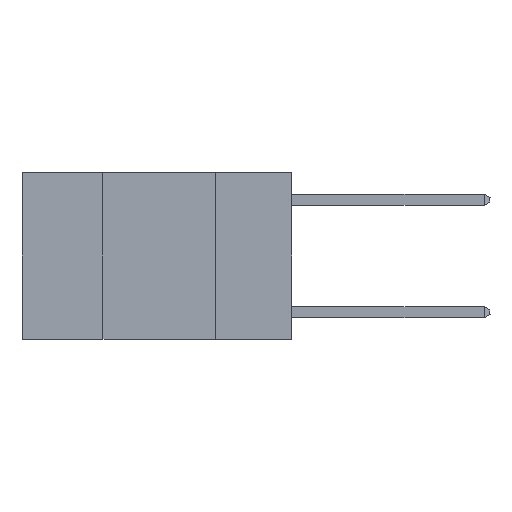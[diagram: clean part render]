
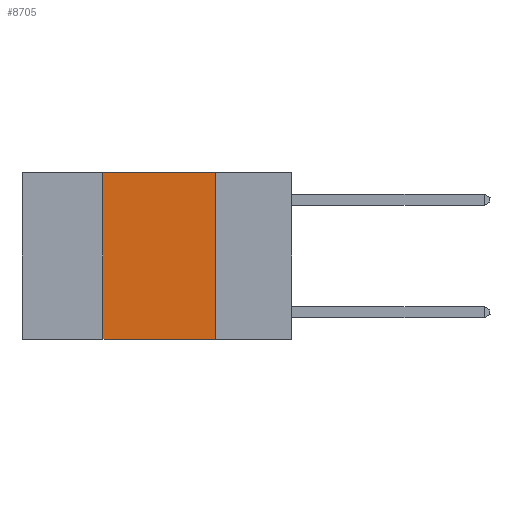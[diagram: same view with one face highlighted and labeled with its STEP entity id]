
A CAD part, left-side view. The second image highlights one B-rep face of the part: STEP entity #8705.
In plain terms, the highlighted planar face has unit normal (-1, 0, 0).
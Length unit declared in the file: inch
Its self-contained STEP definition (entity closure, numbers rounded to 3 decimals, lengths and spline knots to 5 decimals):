
#57 = VERTEX_POINT ( 'NONE', #1477 ) ;
#763 = EDGE_CURVE ( 'NONE', #57, #2991, #19208, .T. ) ;
#1477 = CARTESIAN_POINT ( 'NONE',  ( 0., 0.42, -0.37 ) ) ;
#1705 = AXIS2_PLACEMENT_3D ( 'NONE', #19868, #19673, #16497 ) ;
#2331 = ORIENTED_EDGE ( 'NONE', *, *, #6382, .T. ) ;
#2991 = VERTEX_POINT ( 'NONE', #6717 ) ;
#3141 = EDGE_LOOP ( 'NONE', ( #3991, #3973, #12207, #2331 ) ) ;
#3901 = VECTOR ( 'NONE', #5227, 39.37008 ) ;
#3973 = ORIENTED_EDGE ( 'NONE', *, *, #10713, .F. ) ;
#3991 = ORIENTED_EDGE ( 'NONE', *, *, #4081, .F. ) ;
#4081 = EDGE_CURVE ( 'NONE', #12759, #8186, #7057, .T. ) ;
#4311 = DIRECTION ( 'NONE',  ( 0., 0., -1. ) ) ;
#5227 = DIRECTION ( 'NONE',  ( 0., -1., 0. ) ) ;
#5976 = DIRECTION ( 'NONE',  ( 0., -1., 0. ) ) ;
#6382 = EDGE_CURVE ( 'NONE', #57, #8186, #9386, .T. ) ;
#6596 = VECTOR ( 'NONE', #4311, 39.37008 ) ;
#6717 = CARTESIAN_POINT ( 'NONE',  ( 0., 0.42, 0. ) ) ;
#6753 = LINE ( 'NONE', #19111, #3901 ) ;
#7057 = LINE ( 'NONE', #13520, #6596 ) ;
#8186 = VERTEX_POINT ( 'NONE', #9035 ) ;
#8705 = ADVANCED_FACE ( 'NONE', ( #16796 ), #10626, .F. ) ;
#8751 = DIRECTION ( 'NONE',  ( 0., 0., 1. ) ) ;
#9035 = CARTESIAN_POINT ( 'NONE',  ( 0., 0.17, -0.37 ) ) ;
#9386 = LINE ( 'NONE', #15561, #16663 ) ;
#10503 = VECTOR ( 'NONE', #8751, 39.37008 ) ;
#10626 = PLANE ( 'NONE',  #1705 ) ;
#10713 = EDGE_CURVE ( 'NONE', #2991, #12759, #6753, .T. ) ;
#12207 = ORIENTED_EDGE ( 'NONE', *, *, #763, .F. ) ;
#12759 = VERTEX_POINT ( 'NONE', #15960 ) ;
#13520 = CARTESIAN_POINT ( 'NONE',  ( 0., 0.17, 0. ) ) ;
#15561 = CARTESIAN_POINT ( 'NONE',  ( 0., 0.6, -0.37 ) ) ;
#15960 = CARTESIAN_POINT ( 'NONE',  ( 0., 0.17, 0. ) ) ;
#16497 = DIRECTION ( 'NONE',  ( 0., 0., -1. ) ) ;
#16663 = VECTOR ( 'NONE', #5976, 39.37008 ) ;
#16796 = FACE_OUTER_BOUND ( 'NONE', #3141, .T. ) ;
#19111 = CARTESIAN_POINT ( 'NONE',  ( 0., 0.6, 0. ) ) ;
#19208 = LINE ( 'NONE', #19612, #10503 ) ;
#19612 = CARTESIAN_POINT ( 'NONE',  ( 0., 0.42, 0. ) ) ;
#19673 = DIRECTION ( 'NONE',  ( 1., 0., 0. ) ) ;
#19868 = CARTESIAN_POINT ( 'NONE',  ( 0., 0.6, 0. ) ) ;
